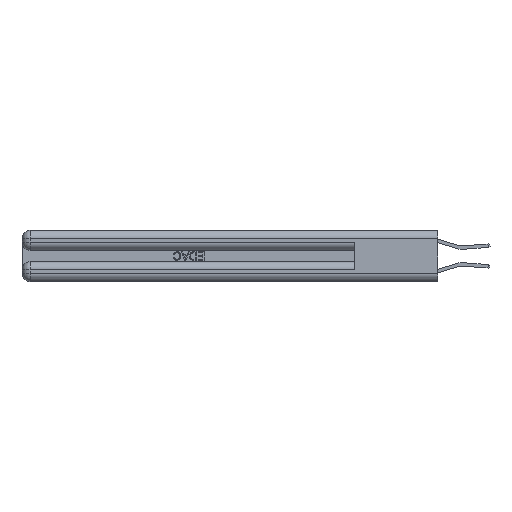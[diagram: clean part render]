
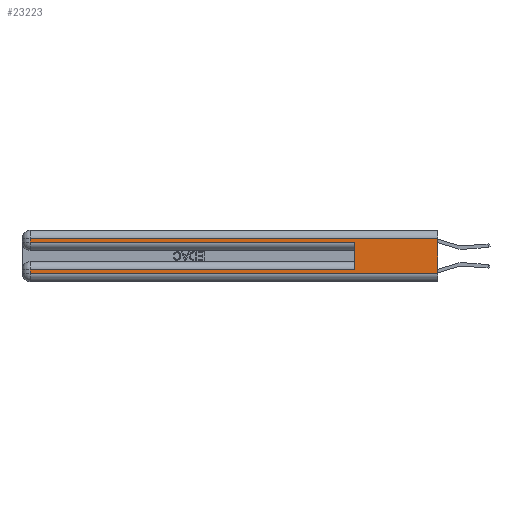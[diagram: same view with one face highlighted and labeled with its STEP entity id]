
A CAD part, left-side view. The second image highlights one B-rep face of the part: STEP entity #23223.
In plain terms, the highlighted planar face has unit normal (-1, 0, 0).
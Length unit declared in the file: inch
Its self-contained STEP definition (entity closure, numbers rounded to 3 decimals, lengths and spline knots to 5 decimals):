
#501 = EDGE_CURVE ( 'NONE', #21362, #7403, #11695, .T. ) ;
#727 = LINE ( 'NONE', #25616, #23325 ) ;
#1077 = EDGE_LOOP ( 'NONE', ( #3843, #22021, #7864, #16277, #15269, #4553, #3407, #23196 ) ) ;
#1106 = VECTOR ( 'NONE', #9657, 39.37008 ) ;
#1304 = CARTESIAN_POINT ( 'NONE',  ( 0., 2.94, 0.37 ) ) ;
#1825 = DIRECTION ( 'NONE',  ( 0., -1., 0. ) ) ;
#2208 = CARTESIAN_POINT ( 'NONE',  ( 0., 0., 0.06 ) ) ;
#2906 = LINE ( 'NONE', #7722, #21836 ) ;
#3324 = CARTESIAN_POINT ( 'NONE',  ( 0., 0., 0.085 ) ) ;
#3407 = ORIENTED_EDGE ( 'NONE', *, *, #15082, .T. ) ;
#3491 = LINE ( 'NONE', #22973, #17444 ) ;
#3843 = ORIENTED_EDGE ( 'NONE', *, *, #15596, .F. ) ;
#4148 = AXIS2_PLACEMENT_3D ( 'NONE', #5274, #9544, #7412 ) ;
#4362 = DIRECTION ( 'NONE',  ( 0., -1., 0. ) ) ;
#4553 = ORIENTED_EDGE ( 'NONE', *, *, #501, .T. ) ;
#4814 = CARTESIAN_POINT ( 'NONE',  ( 0., 2.94, 0.06 ) ) ;
#5274 = CARTESIAN_POINT ( 'NONE',  ( 0., 0., 0.37 ) ) ;
#5790 = FACE_OUTER_BOUND ( 'NONE', #1077, .T. ) ;
#7403 = VERTEX_POINT ( 'NONE', #9129 ) ;
#7412 = DIRECTION ( 'NONE',  ( 0., 0., -1. ) ) ;
#7480 = LINE ( 'NONE', #14443, #13761 ) ;
#7722 = CARTESIAN_POINT ( 'NONE',  ( 0., 0.6, 0.145 ) ) ;
#7864 = ORIENTED_EDGE ( 'NONE', *, *, #16681, .T. ) ;
#8404 = VECTOR ( 'NONE', #11117, 39.37008 ) ;
#9129 = CARTESIAN_POINT ( 'NONE',  ( 0., 2.94, 0.085 ) ) ;
#9434 = CARTESIAN_POINT ( 'NONE',  ( 0., 0., 0.31 ) ) ;
#9453 = VERTEX_POINT ( 'NONE', #27218 ) ;
#9544 = DIRECTION ( 'NONE',  ( 1., 0., 0. ) ) ;
#9657 = DIRECTION ( 'NONE',  ( 0., 0., -1. ) ) ;
#9815 = VERTEX_POINT ( 'NONE', #2208 ) ;
#9835 = DIRECTION ( 'NONE',  ( 0., 0., -1. ) ) ;
#10016 = VERTEX_POINT ( 'NONE', #20687 ) ;
#10293 = CARTESIAN_POINT ( 'NONE',  ( 0., 0.6, 0.085 ) ) ;
#11117 = DIRECTION ( 'NONE',  ( 0., 1., 0. ) ) ;
#11211 = CARTESIAN_POINT ( 'NONE',  ( 0., 0., 0.31 ) ) ;
#11299 = PLANE ( 'NONE',  #4148 ) ;
#11322 = EDGE_CURVE ( 'NONE', #23091, #9815, #727, .T. ) ;
#11440 = EDGE_CURVE ( 'NONE', #21804, #9453, #21978, .T. ) ;
#11695 = LINE ( 'NONE', #3324, #12351 ) ;
#11874 = EDGE_CURVE ( 'NONE', #18487, #10016, #23002, .T. ) ;
#12351 = VECTOR ( 'NONE', #18571, 39.37008 ) ;
#13721 = CARTESIAN_POINT ( 'NONE',  ( 0., 2.94, 0.285 ) ) ;
#13761 = VECTOR ( 'NONE', #9835, 39.37008 ) ;
#14443 = CARTESIAN_POINT ( 'NONE',  ( 0., 0., 0.37 ) ) ;
#15082 = EDGE_CURVE ( 'NONE', #7403, #23091, #3491, .T. ) ;
#15269 = ORIENTED_EDGE ( 'NONE', *, *, #20788, .F. ) ;
#15596 = EDGE_CURVE ( 'NONE', #21804, #9815, #7480, .T. ) ;
#16136 = DIRECTION ( 'NONE',  ( 0., 0., 1. ) ) ;
#16277 = ORIENTED_EDGE ( 'NONE', *, *, #11874, .T. ) ;
#16681 = EDGE_CURVE ( 'NONE', #9453, #18487, #16698, .T. ) ;
#16698 = LINE ( 'NONE', #1304, #1106 ) ;
#17444 = VECTOR ( 'NONE', #25015, 39.37008 ) ;
#18487 = VERTEX_POINT ( 'NONE', #13721 ) ;
#18571 = DIRECTION ( 'NONE',  ( 0., 1., 0. ) ) ;
#20687 = CARTESIAN_POINT ( 'NONE',  ( 0., 0.6, 0.285 ) ) ;
#20788 = EDGE_CURVE ( 'NONE', #21362, #10016, #2906, .T. ) ;
#21362 = VERTEX_POINT ( 'NONE', #10293 ) ;
#21804 = VERTEX_POINT ( 'NONE', #9434 ) ;
#21836 = VECTOR ( 'NONE', #16136, 39.37008 ) ;
#21978 = LINE ( 'NONE', #11211, #8404 ) ;
#22021 = ORIENTED_EDGE ( 'NONE', *, *, #11440, .T. ) ;
#22973 = CARTESIAN_POINT ( 'NONE',  ( 0., 2.94, 0.37 ) ) ;
#23002 = LINE ( 'NONE', #27267, #26631 ) ;
#23091 = VERTEX_POINT ( 'NONE', #4814 ) ;
#23196 = ORIENTED_EDGE ( 'NONE', *, *, #11322, .T. ) ;
#23223 = ADVANCED_FACE ( 'NONE', ( #5790 ), #11299, .F. ) ;
#23325 = VECTOR ( 'NONE', #4362, 39.37008 ) ;
#25015 = DIRECTION ( 'NONE',  ( 0., 0., -1. ) ) ;
#25616 = CARTESIAN_POINT ( 'NONE',  ( 0., 0., 0.06 ) ) ;
#26631 = VECTOR ( 'NONE', #1825, 39.37008 ) ;
#27218 = CARTESIAN_POINT ( 'NONE',  ( 0., 2.94, 0.31 ) ) ;
#27267 = CARTESIAN_POINT ( 'NONE',  ( 0., 0., 0.285 ) ) ;
